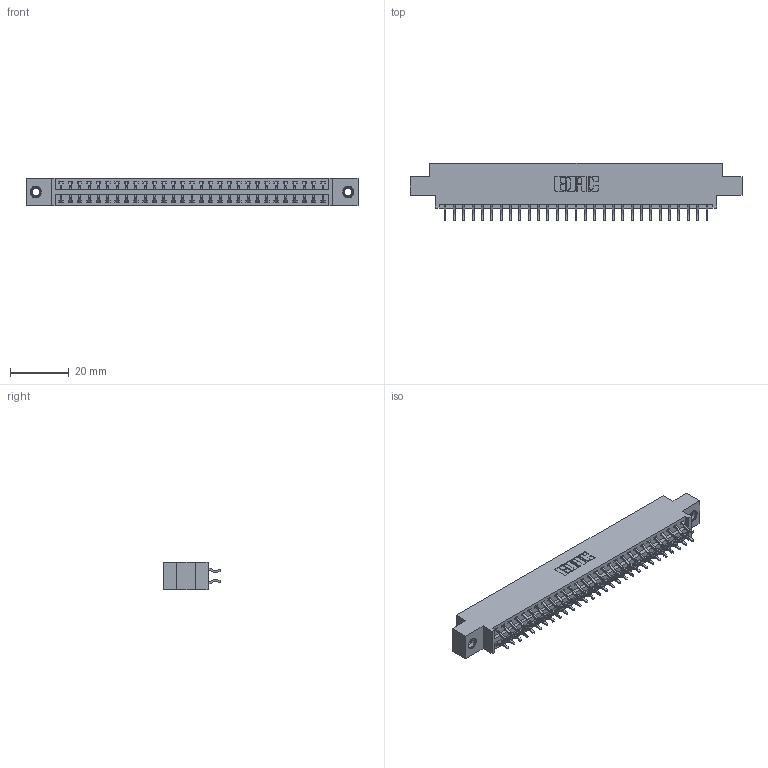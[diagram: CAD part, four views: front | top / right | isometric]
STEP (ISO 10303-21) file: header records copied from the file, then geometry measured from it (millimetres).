
FILE_DESCRIPTION (( 'STEP AP203' ), '1' );
FILE_NAME ('346-058-556-807.STEP', '2022-05-21T09:14:54', ( '' ), ( '' ), 'SwSTEP 2.0', 'SolidWorks 2020', '' );
FILE_SCHEMA (( 'CONFIG_CONTROL_DESIGN' ));
Length unit declared in the file: inch
Products named in the file (4): 346 Part_0.170 Offset - 0.156 Dia-TI; 345-250-001_345-250-005-103; 345-292-001_556 Tail; 346-058-556-807
Assembly tree (61 placements, depth 2):
  346-058-556-807
    346 Part_0.170 Offset - 0.156 Dia-TI
    345-292-001_556 Tail  x58
    345-250-001_345-250-005-103  x2
Bounding box: 112.65 x 19.57 x 9.4 mm (x, y, z)
Volume: 10713.3 mm3; surface area: 14681.3 mm2
Topology: 61 solids, 61 shells, 3550 faces, 10511 edges, 6922 vertices
Faces by surface type: plane 2374, cylinder 1160, cone 12, torus 4
Entity records: 22214 total; most frequent: CARTESIAN_POINT 3679, ORIENTED_EDGE 3594, DIRECTION 3307, EDGE_CURVE 1797, VECTOR 1521, LINE 1521, VERTEX_POINT 1192, AXIS2_PLACEMENT_3D 893
